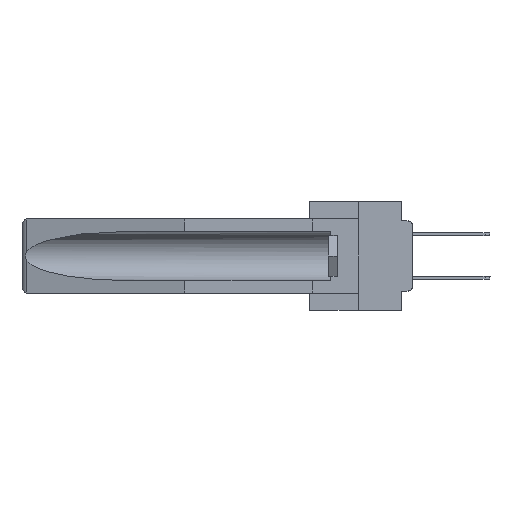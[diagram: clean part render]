
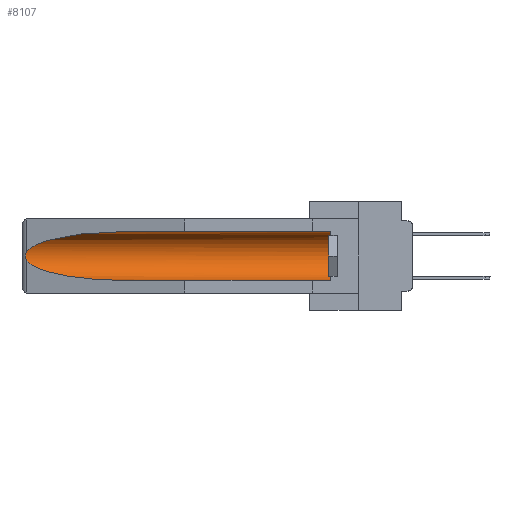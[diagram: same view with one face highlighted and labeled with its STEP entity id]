
A CAD part, left-side view. The second image highlights one B-rep face of the part: STEP entity #8107.
In plain terms, the highlighted cylindrical face has radius 2.857 mm (diameter 5.715 mm), a partial arc.
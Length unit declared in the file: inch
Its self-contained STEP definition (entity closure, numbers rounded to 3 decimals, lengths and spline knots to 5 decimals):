
#99 = CARTESIAN_POINT ( 'NONE',  ( 0.155, 0.126, -0.1715 ) ) ;
#459 = CARTESIAN_POINT ( 'NONE',  ( 0.155, 1.07973, -0.284 ) ) ;
#1034 = CARTESIAN_POINT ( 'NONE',  ( 0.25451, 1.48313, -0.24835 ) ) ;
#1433 = CARTESIAN_POINT ( 'NONE',  ( 0.155, 0.126, -0.059 ) ) ;
#3369 = CARTESIAN_POINT ( 'NONE',  ( 0.26537, 1.52718, -0.19328 ) ) ;
#3736 = CIRCLE ( 'NONE', #6203, 0.1125 ) ;
#4498 = VERTEX_POINT ( 'NONE', #1433 ) ;
#6203 = AXIS2_PLACEMENT_3D ( 'NONE', #99, #17747, #14651 ) ;
#6892 = EDGE_CURVE ( 'NONE', #34745, #30713, #12591, .T. ) ;
#7681 = CARTESIAN_POINT ( 'NONE',  ( 0.26655, 1.53094, -0.18657 ) ) ;
#8107 = ADVANCED_FACE ( 'NONE', ( #24648 ), #35714, .F. ) ;
#8779 = CARTESIAN_POINT ( 'NONE',  ( 0.155, 1.07973, -0.059 ) ) ;
#9205 = CARTESIAN_POINT ( 'NONE',  ( 0.155, -0.30754, -0.1715 ) ) ;
#9846 = VERTEX_POINT ( 'NONE', #33716 ) ;
#10383 = CARTESIAN_POINT ( 'NONE',  ( 0.2673, 1.5327, -0.16383 ) ) ;
#12591 = B_SPLINE_CURVE_WITH_KNOTS ( 'NONE', 3,
 ( #33817, #25646, #19853, #10383, #37279, #33995, #27959, #7681, #31677, #22758 ),
 .UNSPECIFIED., .F., .F.,
 ( 4, 2, 2, 2, 4 ),
 ( 0., 0.00029, 0.00058, 0.00087, 0.00117 ),
 .UNSPECIFIED. ) ;
#12989 = EDGE_CURVE ( 'NONE', #30713, #13446, #22648, .T. ) ;
#12999 = ORIENTED_EDGE ( 'NONE', *, *, #37801, .F. ) ;
#13271 =( BOUNDED_CURVE ( )  B_SPLINE_CURVE ( 3, ( #32794, #24444, #24056, #35875 ),
 .UNSPECIFIED., .F., .F. ) 
 B_SPLINE_CURVE_WITH_KNOTS ( ( 4, 4 ),
 ( 4.71239, 6.08839 ),
 .UNSPECIFIED. ) 
 CURVE ( )  GEOMETRIC_REPRESENTATION_ITEM ( )  RATIONAL_B_SPLINE_CURVE ( ( 1., 0.848, 0.848, 1. ) ) 
 REPRESENTATION_ITEM ( '' )  );
#13446 = VERTEX_POINT ( 'NONE', #22206 ) ;
#13910 = CARTESIAN_POINT ( 'NONE',  ( 0.155, -0.30754, -0.284 ) ) ;
#14651 = DIRECTION ( 'NONE',  ( 0., 0., 1. ) ) ;
#15081 = AXIS2_PLACEMENT_3D ( 'NONE', #9205, #35897, #27333 ) ;
#16918 = CARTESIAN_POINT ( 'NONE',  ( 0.155, -0.30754, -0.059 ) ) ;
#17747 = DIRECTION ( 'NONE',  ( 0., -1., 0. ) ) ;
#17838 = EDGE_LOOP ( 'NONE', ( #23519, #19894, #36569, #12999, #26676, #26829 ) ) ;
#18917 = VERTEX_POINT ( 'NONE', #8779 ) ;
#19853 = CARTESIAN_POINT ( 'NONE',  ( 0.26654, 1.53092, -0.15636 ) ) ;
#19894 = ORIENTED_EDGE ( 'NONE', *, *, #6892, .T. ) ;
#19899 = LINE ( 'NONE', #13910, #23629 ) ;
#20036 = EDGE_CURVE ( 'NONE', #4498, #18917, #22903, .T. ) ;
#22206 = CARTESIAN_POINT ( 'NONE',  ( 0.155, 1.07973, -0.284 ) ) ;
#22648 =( BOUNDED_CURVE ( )  B_SPLINE_CURVE ( 3, ( #3369, #1034, #33377, #459 ),
 .UNSPECIFIED., .F., .T. ) 
 B_SPLINE_CURVE_WITH_KNOTS ( ( 4, 4 ),
 ( 0.1948, 1.5708 ),
 .UNSPECIFIED. ) 
 CURVE ( )  GEOMETRIC_REPRESENTATION_ITEM ( )  RATIONAL_B_SPLINE_CURVE ( ( 1., 0.848, 0.848, 1. ) ) 
 REPRESENTATION_ITEM ( '' )  );
#22758 = CARTESIAN_POINT ( 'NONE',  ( 0.26537, 1.52718, -0.19328 ) ) ;
#22903 = LINE ( 'NONE', #16918, #24406 ) ;
#23519 = ORIENTED_EDGE ( 'NONE', *, *, #30286, .T. ) ;
#23629 = VECTOR ( 'NONE', #34439, 39.37008 ) ;
#24056 = CARTESIAN_POINT ( 'NONE',  ( 0.25451, 1.48313, -0.09465 ) ) ;
#24392 = EDGE_CURVE ( 'NONE', #9846, #4498, #3736, .T. ) ;
#24406 = VECTOR ( 'NONE', #25968, 39.37008 ) ;
#24444 = CARTESIAN_POINT ( 'NONE',  ( 0.21114, 1.30732, -0.059 ) ) ;
#24648 = FACE_OUTER_BOUND ( 'NONE', #17838, .T. ) ;
#25646 = CARTESIAN_POINT ( 'NONE',  ( 0.26597, 1.52961, -0.15275 ) ) ;
#25968 = DIRECTION ( 'NONE',  ( 0., 1., 0. ) ) ;
#26676 = ORIENTED_EDGE ( 'NONE', *, *, #24392, .T. ) ;
#26829 = ORIENTED_EDGE ( 'NONE', *, *, #20036, .T. ) ;
#27333 = DIRECTION ( 'NONE',  ( 0., 0., 1. ) ) ;
#27959 = CARTESIAN_POINT ( 'NONE',  ( 0.2673, 1.53269, -0.17917 ) ) ;
#29108 = CARTESIAN_POINT ( 'NONE',  ( 0.26537, 1.52718, -0.14972 ) ) ;
#30286 = EDGE_CURVE ( 'NONE', #18917, #34745, #13271, .T. ) ;
#30713 = VERTEX_POINT ( 'NONE', #35836 ) ;
#31677 = CARTESIAN_POINT ( 'NONE',  ( 0.26597, 1.5296, -0.19026 ) ) ;
#32794 = CARTESIAN_POINT ( 'NONE',  ( 0.155, 1.07973, -0.059 ) ) ;
#33377 = CARTESIAN_POINT ( 'NONE',  ( 0.21114, 1.30732, -0.284 ) ) ;
#33716 = CARTESIAN_POINT ( 'NONE',  ( 0.155, 0.126, -0.284 ) ) ;
#33817 = CARTESIAN_POINT ( 'NONE',  ( 0.26537, 1.52718, -0.14972 ) ) ;
#33995 = CARTESIAN_POINT ( 'NONE',  ( 0.2675, 1.53308, -0.17534 ) ) ;
#34439 = DIRECTION ( 'NONE',  ( 0., 1., 0. ) ) ;
#34745 = VERTEX_POINT ( 'NONE', #29108 ) ;
#35714 = CYLINDRICAL_SURFACE ( 'NONE', #15081, 0.1125 ) ;
#35836 = CARTESIAN_POINT ( 'NONE',  ( 0.26537, 1.52718, -0.19328 ) ) ;
#35875 = CARTESIAN_POINT ( 'NONE',  ( 0.26537, 1.52718, -0.14972 ) ) ;
#35897 = DIRECTION ( 'NONE',  ( 0., 1., 0. ) ) ;
#36569 = ORIENTED_EDGE ( 'NONE', *, *, #12989, .T. ) ;
#37279 = CARTESIAN_POINT ( 'NONE',  ( 0.2675, 1.53308, -0.16763 ) ) ;
#37801 = EDGE_CURVE ( 'NONE', #9846, #13446, #19899, .T. ) ;
